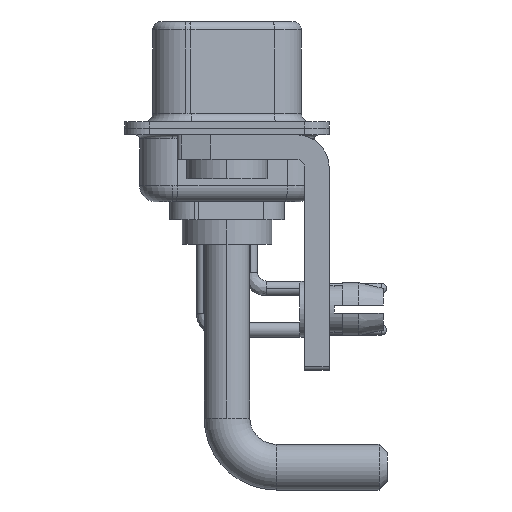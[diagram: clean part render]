
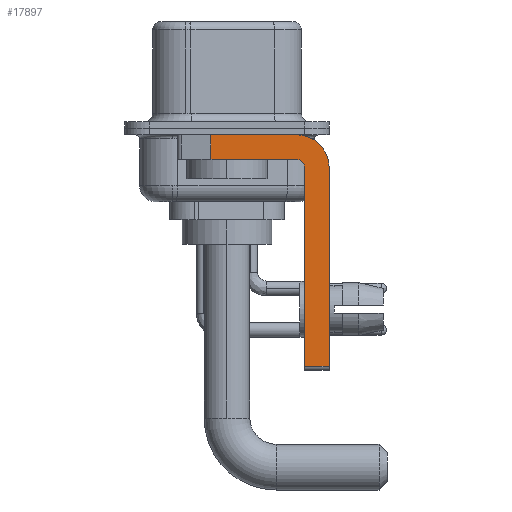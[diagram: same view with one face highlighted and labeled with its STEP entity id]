
A CAD part, left-side view. The second image highlights one B-rep face of the part: STEP entity #17897.
In plain terms, the highlighted planar face has unit normal (-1, 0, 0).
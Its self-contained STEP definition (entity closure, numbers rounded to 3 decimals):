
#331 = AXIS2_PLACEMENT_3D ( 'NONE', #6629, #22816, #20436 ) ;
#650 = VERTEX_POINT ( 'NONE', #25405 ) ;
#1214 = VERTEX_POINT ( 'NONE', #7383 ) ;
#1389 = VERTEX_POINT ( 'NONE', #28585 ) ;
#1439 = VERTEX_POINT ( 'NONE', #9520 ) ;
#1528 = DIRECTION ( 'NONE',  ( 0., 0., 1. ) ) ;
#1863 = FACE_OUTER_BOUND ( 'NONE', #24947, .T. ) ;
#2375 = DIRECTION ( 'NONE',  ( 1., 0., 0. ) ) ;
#2590 = VECTOR ( 'NONE', #1528, 1000. ) ;
#2951 = ORIENTED_EDGE ( 'NONE', *, *, #23698, .F. ) ;
#3301 = VECTOR ( 'NONE', #11361, 1000. ) ;
#3537 = CARTESIAN_POINT ( 'NONE',  ( -2.9, -4.25, -0.4 ) ) ;
#3550 = LINE ( 'NONE', #27927, #28496 ) ;
#4678 = CARTESIAN_POINT ( 'NONE',  ( -2.9, 0.978, -1.9 ) ) ;
#5208 = LINE ( 'NONE', #19018, #17473 ) ;
#5454 = CARTESIAN_POINT ( 'NONE',  ( -2.9, -4.25, -14.55 ) ) ;
#5798 = DIRECTION ( 'NONE',  ( 0., 0., -1. ) ) ;
#5988 = CARTESIAN_POINT ( 'NONE',  ( -2.9, -4.75, -14.8 ) ) ;
#6052 = CIRCLE ( 'NONE', #331, 0.5 ) ;
#6159 = ORIENTED_EDGE ( 'NONE', *, *, #14708, .T. ) ;
#6405 = LINE ( 'NONE', #26751, #21379 ) ;
#6629 = CARTESIAN_POINT ( 'NONE',  ( -2.9, -4.25, -2.4 ) ) ;
#6652 = VERTEX_POINT ( 'NONE', #4678 ) ;
#7383 = CARTESIAN_POINT ( 'NONE',  ( -2.9, -6.25, -14.55 ) ) ;
#7599 = DIRECTION ( 'NONE',  ( 0., 0., -1. ) ) ;
#8080 = LINE ( 'NONE', #5988, #2590 ) ;
#8895 = EDGE_CURVE ( 'NONE', #27142, #1439, #22287, .T. ) ;
#9082 = DIRECTION ( 'NONE',  ( 0., 0., -1. ) ) ;
#9520 = CARTESIAN_POINT ( 'NONE',  ( -2.9, -6.25, -2.4 ) ) ;
#9664 = CARTESIAN_POINT ( 'NONE',  ( -2.9, -4.25, -2.4 ) ) ;
#10538 = EDGE_CURVE ( 'NONE', #1439, #1214, #3550, .T. ) ;
#10954 = VERTEX_POINT ( 'NONE', #21208 ) ;
#11361 = DIRECTION ( 'NONE',  ( 0., 1., 0. ) ) ;
#11851 = DIRECTION ( 'NONE',  ( 0., -1., 0. ) ) ;
#12764 = VECTOR ( 'NONE', #11851, 1000. ) ;
#13293 = AXIS2_PLACEMENT_3D ( 'NONE', #9664, #2375, #9082 ) ;
#14708 = EDGE_CURVE ( 'NONE', #10954, #6652, #5208, .T. ) ;
#15228 = EDGE_CURVE ( 'NONE', #15450, #1214, #25669, .T. ) ;
#15394 = CARTESIAN_POINT ( 'NONE',  ( -2.9, -4.25, -2.4 ) ) ;
#15450 = VERTEX_POINT ( 'NONE', #19918 ) ;
#15484 = ORIENTED_EDGE ( 'NONE', *, *, #27836, .F. ) ;
#15732 = ORIENTED_EDGE ( 'NONE', *, *, #16096, .F. ) ;
#16096 = EDGE_CURVE ( 'NONE', #650, #6652, #27106, .T. ) ;
#16863 = EDGE_CURVE ( 'NONE', #10954, #27142, #6405, .T. ) ;
#17473 = VECTOR ( 'NONE', #5798, 1000. ) ;
#17897 = ADVANCED_FACE ( 'NONE', ( #1863 ), #19998, .F. ) ;
#18062 = DIRECTION ( 'NONE',  ( 0., 0., -1. ) ) ;
#18296 = ORIENTED_EDGE ( 'NONE', *, *, #8895, .F. ) ;
#19018 = CARTESIAN_POINT ( 'NONE',  ( -2.9, 0.978, -1.9 ) ) ;
#19783 = ORIENTED_EDGE ( 'NONE', *, *, #10538, .F. ) ;
#19918 = CARTESIAN_POINT ( 'NONE',  ( -2.9, -4.75, -14.55 ) ) ;
#19998 = PLANE ( 'NONE',  #24724 ) ;
#20426 = CARTESIAN_POINT ( 'NONE',  ( -2.9, -4.25, -1.9 ) ) ;
#20436 = DIRECTION ( 'NONE',  ( 0., 0., 1. ) ) ;
#21208 = CARTESIAN_POINT ( 'NONE',  ( -2.9, 0.978, -0.4 ) ) ;
#21379 = VECTOR ( 'NONE', #28805, 1000. ) ;
#21960 = ORIENTED_EDGE ( 'NONE', *, *, #15228, .T. ) ;
#22287 = CIRCLE ( 'NONE', #13293, 2. ) ;
#22507 = DIRECTION ( 'NONE',  ( 1., 0., 0. ) ) ;
#22816 = DIRECTION ( 'NONE',  ( -1., 0., 0. ) ) ;
#23698 = EDGE_CURVE ( 'NONE', #15450, #1389, #8080, .T. ) ;
#24724 = AXIS2_PLACEMENT_3D ( 'NONE', #15394, #22507, #18062 ) ;
#24947 = EDGE_LOOP ( 'NONE', ( #25217, #6159, #15732, #15484, #2951, #21960, #19783, #18296 ) ) ;
#25217 = ORIENTED_EDGE ( 'NONE', *, *, #16863, .F. ) ;
#25405 = CARTESIAN_POINT ( 'NONE',  ( -2.9, -4.25, -1.9 ) ) ;
#25669 = LINE ( 'NONE', #5454, #12764 ) ;
#26751 = CARTESIAN_POINT ( 'NONE',  ( -2.9, 3., -0.4 ) ) ;
#27106 = LINE ( 'NONE', #20426, #3301 ) ;
#27142 = VERTEX_POINT ( 'NONE', #3537 ) ;
#27836 = EDGE_CURVE ( 'NONE', #1389, #650, #6052, .T. ) ;
#27927 = CARTESIAN_POINT ( 'NONE',  ( -2.9, -6.25, -2.4 ) ) ;
#28496 = VECTOR ( 'NONE', #7599, 1000. ) ;
#28585 = CARTESIAN_POINT ( 'NONE',  ( -2.9, -4.75, -2.4 ) ) ;
#28805 = DIRECTION ( 'NONE',  ( 0., -1., 0. ) ) ;
